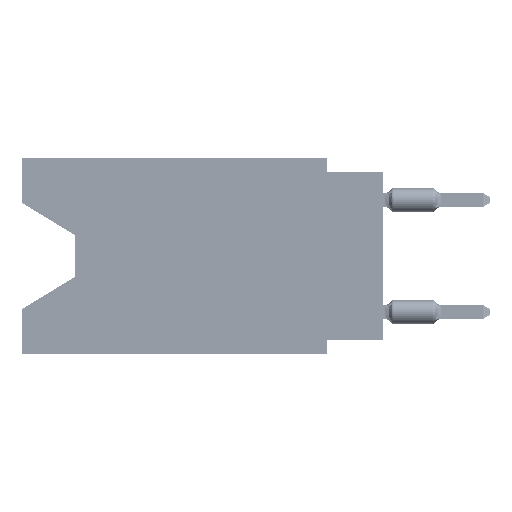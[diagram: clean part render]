
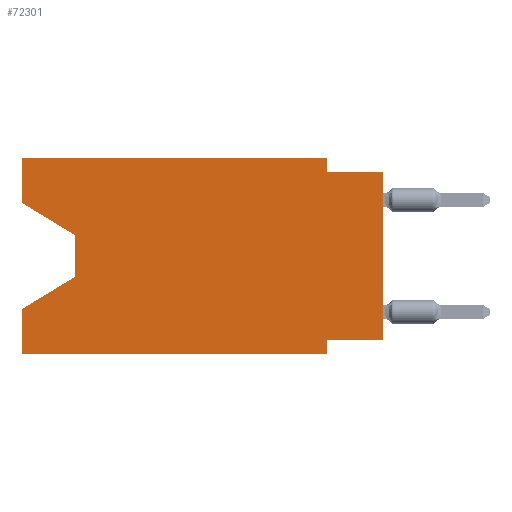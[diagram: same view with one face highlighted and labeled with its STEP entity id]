
A CAD part, left-side view. The second image highlights one B-rep face of the part: STEP entity #72301.
In plain terms, the highlighted planar face has unit normal (-1, 0, 0).
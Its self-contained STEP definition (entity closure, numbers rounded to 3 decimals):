
#111 = CARTESIAN_POINT ( 'NONE',  ( 0., 0., -0.635 ) ) ;
#1134 = ORIENTED_EDGE ( 'NONE', *, *, #48288, .T. ) ;
#5095 = VERTEX_POINT ( 'NONE', #52417 ) ;
#5148 = VECTOR ( 'NONE', #46444, 1000. ) ;
#5602 = LINE ( 'NONE', #59402, #47856 ) ;
#5835 = LINE ( 'NONE', #73174, #12864 ) ;
#7648 = EDGE_CURVE ( 'NONE', #66898, #51203, #5835, .T. ) ;
#8126 = DIRECTION ( 'NONE',  ( 0., 1., 0. ) ) ;
#11373 = CARTESIAN_POINT ( 'NONE',  ( 0., 16.383, 0. ) ) ;
#12864 = VECTOR ( 'NONE', #29746, 1000. ) ;
#17534 = DIRECTION ( 'NONE',  ( 0., 0., -1. ) ) ;
#18689 = LINE ( 'NONE', #47789, #62121 ) ;
#19370 = CARTESIAN_POINT ( 'NONE',  ( 0., 2.54, -8.255 ) ) ;
#19832 = FACE_OUTER_BOUND ( 'NONE', #23889, .T. ) ;
#21647 = VERTEX_POINT ( 'NONE', #59313 ) ;
#23725 = EDGE_CURVE ( 'NONE', #72144, #71932, #78738, .T. ) ;
#23889 = EDGE_LOOP ( 'NONE', ( #1134, #34947, #25034, #57291, #63476, #26940, #47924, #29099, #34798, #27848, #61831, #43564 ) ) ;
#24143 = DIRECTION ( 'NONE',  ( 0., -1., 0. ) ) ;
#24190 = VECTOR ( 'NONE', #76269, 1000. ) ;
#24338 = DIRECTION ( 'NONE',  ( 0., 0., -1. ) ) ;
#25034 = ORIENTED_EDGE ( 'NONE', *, *, #64539, .T. ) ;
#25158 = VERTEX_POINT ( 'NONE', #19370 ) ;
#25401 = LINE ( 'NONE', #38146, #24190 ) ;
#26507 = VERTEX_POINT ( 'NONE', #75280 ) ;
#26940 = ORIENTED_EDGE ( 'NONE', *, *, #35703, .F. ) ;
#27374 = EDGE_CURVE ( 'NONE', #26507, #51203, #5602, .T. ) ;
#27774 = VECTOR ( 'NONE', #32404, 1000. ) ;
#27848 = ORIENTED_EDGE ( 'NONE', *, *, #65305, .F. ) ;
#29012 = CARTESIAN_POINT ( 'NONE',  ( 0., 16.383, -6.852 ) ) ;
#29099 = ORIENTED_EDGE ( 'NONE', *, *, #7648, .T. ) ;
#29536 = DIRECTION ( 'NONE',  ( 1., 0., 0. ) ) ;
#29691 = LINE ( 'NONE', #11373, #5148 ) ;
#29746 = DIRECTION ( 'NONE',  ( 0., 0., 1. ) ) ;
#30313 = PLANE ( 'NONE',  #73370 ) ;
#30500 = LINE ( 'NONE', #54014, #62986 ) ;
#30728 = CARTESIAN_POINT ( 'NONE',  ( 0., 13.97, -3.505 ) ) ;
#30807 = CARTESIAN_POINT ( 'NONE',  ( 0., 2.54, -8.89 ) ) ;
#31115 = CARTESIAN_POINT ( 'NONE',  ( 0., 2.54, 0. ) ) ;
#32404 = DIRECTION ( 'NONE',  ( 0., -0.855, -0.519 ) ) ;
#33360 = EDGE_CURVE ( 'NONE', #38303, #5095, #78159, .T. ) ;
#33507 = VERTEX_POINT ( 'NONE', #29012 ) ;
#34153 = EDGE_CURVE ( 'NONE', #72401, #45528, #29691, .T. ) ;
#34798 = ORIENTED_EDGE ( 'NONE', *, *, #27374, .F. ) ;
#34947 = ORIENTED_EDGE ( 'NONE', *, *, #33360, .T. ) ;
#35703 = EDGE_CURVE ( 'NONE', #25158, #71932, #25401, .T. ) ;
#36091 = CARTESIAN_POINT ( 'NONE',  ( 0., 16.383, -8.89 ) ) ;
#38146 = CARTESIAN_POINT ( 'NONE',  ( 0., 2.54, -8.89 ) ) ;
#38303 = VERTEX_POINT ( 'NONE', #68531 ) ;
#38462 = VECTOR ( 'NONE', #60375, 1000. ) ;
#41485 = CARTESIAN_POINT ( 'NONE',  ( 0., 16.383, -8.89 ) ) ;
#43254 = CARTESIAN_POINT ( 'NONE',  ( 0., 16.383, 0. ) ) ;
#43564 = ORIENTED_EDGE ( 'NONE', *, *, #55198, .F. ) ;
#45528 = VERTEX_POINT ( 'NONE', #31115 ) ;
#45707 = CARTESIAN_POINT ( 'NONE',  ( 0., 16.383, 0. ) ) ;
#46341 = VECTOR ( 'NONE', #24143, 1000. ) ;
#46444 = DIRECTION ( 'NONE',  ( 0., -1., 0. ) ) ;
#46655 = LINE ( 'NONE', #59002, #66757 ) ;
#47639 = DIRECTION ( 'NONE',  ( 0., 0.855, -0.519 ) ) ;
#47789 = CARTESIAN_POINT ( 'NONE',  ( 0., 16.383, 0. ) ) ;
#47856 = VECTOR ( 'NONE', #66567, 1000. ) ;
#47924 = ORIENTED_EDGE ( 'NONE', *, *, #70342, .F. ) ;
#48288 = EDGE_CURVE ( 'NONE', #21647, #38303, #62299, .T. ) ;
#51203 = VERTEX_POINT ( 'NONE', #111 ) ;
#52417 = CARTESIAN_POINT ( 'NONE',  ( 0., 13.97, -5.385 ) ) ;
#54014 = CARTESIAN_POINT ( 'NONE',  ( 0., 13.97, -5.385 ) ) ;
#55198 = EDGE_CURVE ( 'NONE', #21647, #72401, #18689, .T. ) ;
#55384 = VECTOR ( 'NONE', #17534, 1000. ) ;
#56331 = CARTESIAN_POINT ( 'NONE',  ( 0., 16.383, -2.038 ) ) ;
#57291 = ORIENTED_EDGE ( 'NONE', *, *, #59450, .F. ) ;
#59002 = CARTESIAN_POINT ( 'NONE',  ( 0., 0., -8.255 ) ) ;
#59313 = CARTESIAN_POINT ( 'NONE',  ( 0., 16.383, -2.038 ) ) ;
#59402 = CARTESIAN_POINT ( 'NONE',  ( 0., 0., -0.635 ) ) ;
#59450 = EDGE_CURVE ( 'NONE', #72144, #33507, #66750, .T. ) ;
#60150 = DIRECTION ( 'NONE',  ( 0., 0., 1. ) ) ;
#60375 = DIRECTION ( 'NONE',  ( 0., 0., 1. ) ) ;
#61831 = ORIENTED_EDGE ( 'NONE', *, *, #34153, .F. ) ;
#62121 = VECTOR ( 'NONE', #60150, 1000. ) ;
#62299 = LINE ( 'NONE', #56331, #27774 ) ;
#62453 = CARTESIAN_POINT ( 'NONE',  ( 0., 16.383, 0. ) ) ;
#62986 = VECTOR ( 'NONE', #47639, 1000. ) ;
#63476 = ORIENTED_EDGE ( 'NONE', *, *, #23725, .T. ) ;
#64539 = EDGE_CURVE ( 'NONE', #5095, #33507, #30500, .T. ) ;
#65305 = EDGE_CURVE ( 'NONE', #45528, #26507, #66923, .T. ) ;
#66567 = DIRECTION ( 'NONE',  ( 0., -1., 0. ) ) ;
#66750 = LINE ( 'NONE', #43254, #38462 ) ;
#66757 = VECTOR ( 'NONE', #8126, 1000. ) ;
#66898 = VERTEX_POINT ( 'NONE', #70309 ) ;
#66923 = LINE ( 'NONE', #72121, #55384 ) ;
#68531 = CARTESIAN_POINT ( 'NONE',  ( 0., 13.97, -3.505 ) ) ;
#69995 = VECTOR ( 'NONE', #72974, 1000. ) ;
#70309 = CARTESIAN_POINT ( 'NONE',  ( 0., 0., -8.255 ) ) ;
#70342 = EDGE_CURVE ( 'NONE', #66898, #25158, #46655, .T. ) ;
#71932 = VERTEX_POINT ( 'NONE', #30807 ) ;
#72121 = CARTESIAN_POINT ( 'NONE',  ( 0., 2.54, 0. ) ) ;
#72144 = VERTEX_POINT ( 'NONE', #41485 ) ;
#72301 = ADVANCED_FACE ( 'NONE', ( #19832 ), #30313, .F. ) ;
#72401 = VERTEX_POINT ( 'NONE', #45707 ) ;
#72974 = DIRECTION ( 'NONE',  ( 0., 0., -1. ) ) ;
#73174 = CARTESIAN_POINT ( 'NONE',  ( 0., 0., 0. ) ) ;
#73370 = AXIS2_PLACEMENT_3D ( 'NONE', #62453, #29536, #24338 ) ;
#75280 = CARTESIAN_POINT ( 'NONE',  ( 0., 2.54, -0.635 ) ) ;
#76269 = DIRECTION ( 'NONE',  ( 0., 0., -1. ) ) ;
#78159 = LINE ( 'NONE', #30728, #69995 ) ;
#78738 = LINE ( 'NONE', #36091, #46341 ) ;
